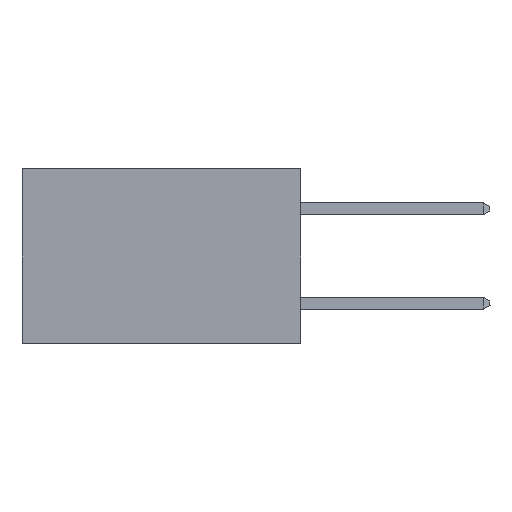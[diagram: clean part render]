
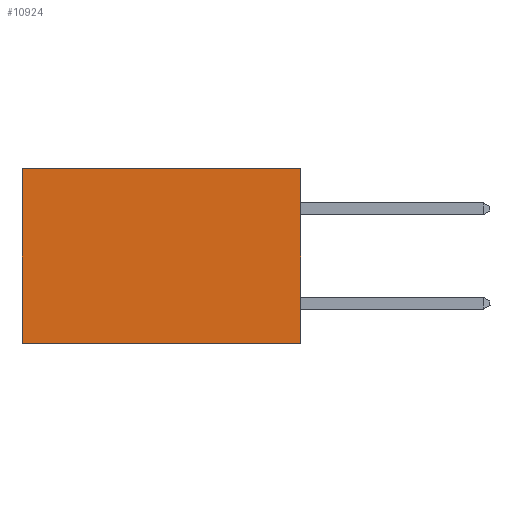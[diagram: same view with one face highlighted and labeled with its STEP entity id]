
A CAD part, left-side view. The second image highlights one B-rep face of the part: STEP entity #10924.
In plain terms, the highlighted planar face has unit normal (-1, 0, 0).
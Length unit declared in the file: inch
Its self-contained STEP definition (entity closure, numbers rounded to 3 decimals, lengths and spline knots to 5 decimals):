
#751 = LINE ( 'NONE', #3941, #12327 ) ;
#842 = EDGE_LOOP ( 'NONE', ( #27502, #11321, #12045, #11987 ) ) ;
#1211 = CARTESIAN_POINT ( 'NONE',  ( 0.277, 0.59, -0.37 ) ) ;
#2899 = DIRECTION ( 'NONE',  ( 0., 0., -1. ) ) ;
#3173 = CARTESIAN_POINT ( 'NONE',  ( 0.277, 0., 0. ) ) ;
#3523 = EDGE_CURVE ( 'NONE', #18295, #16183, #16042, .T. ) ;
#3941 = CARTESIAN_POINT ( 'NONE',  ( 0.277, 0., -0.37 ) ) ;
#4225 = DIRECTION ( 'NONE',  ( 0., 1., 0. ) ) ;
#4241 = DIRECTION ( 'NONE',  ( 0., 0., -1. ) ) ;
#5391 = VECTOR ( 'NONE', #5540, 39.37008 ) ;
#5540 = DIRECTION ( 'NONE',  ( 0., 1., 0. ) ) ;
#6784 = EDGE_CURVE ( 'NONE', #14167, #24368, #751, .T. ) ;
#8692 = PLANE ( 'NONE',  #21738 ) ;
#10018 = VECTOR ( 'NONE', #4225, 39.37008 ) ;
#10924 = ADVANCED_FACE ( 'NONE', ( #20927 ), #8692, .F. ) ;
#11009 = DIRECTION ( 'NONE',  ( 0., 0., -1. ) ) ;
#11321 = ORIENTED_EDGE ( 'NONE', *, *, #28337, .F. ) ;
#11987 = ORIENTED_EDGE ( 'NONE', *, *, #23821, .T. ) ;
#12045 = ORIENTED_EDGE ( 'NONE', *, *, #6784, .F. ) ;
#12327 = VECTOR ( 'NONE', #4241, 39.37008 ) ;
#12391 = CARTESIAN_POINT ( 'NONE',  ( 0.277, 0., -0.37 ) ) ;
#14167 = VERTEX_POINT ( 'NONE', #3173 ) ;
#15190 = CARTESIAN_POINT ( 'NONE',  ( 0.277, 0.59, 0. ) ) ;
#15632 = CARTESIAN_POINT ( 'NONE',  ( 0.277, 0., 0. ) ) ;
#16042 = LINE ( 'NONE', #1211, #20543 ) ;
#16183 = VERTEX_POINT ( 'NONE', #16940 ) ;
#16940 = CARTESIAN_POINT ( 'NONE',  ( 0.277, 0.59, -0.37 ) ) ;
#17332 = CARTESIAN_POINT ( 'NONE',  ( 0.277, 0., -0.37 ) ) ;
#18295 = VERTEX_POINT ( 'NONE', #15190 ) ;
#20543 = VECTOR ( 'NONE', #2899, 39.37008 ) ;
#20927 = FACE_OUTER_BOUND ( 'NONE', #842, .T. ) ;
#21738 = AXIS2_PLACEMENT_3D ( 'NONE', #22126, #24311, #11009 ) ;
#22126 = CARTESIAN_POINT ( 'NONE',  ( 0.277, 0., -0.37 ) ) ;
#23368 = LINE ( 'NONE', #12391, #5391 ) ;
#23821 = EDGE_CURVE ( 'NONE', #14167, #18295, #25669, .T. ) ;
#24311 = DIRECTION ( 'NONE',  ( 1., 0., 0. ) ) ;
#24368 = VERTEX_POINT ( 'NONE', #17332 ) ;
#25669 = LINE ( 'NONE', #15632, #10018 ) ;
#27502 = ORIENTED_EDGE ( 'NONE', *, *, #3523, .T. ) ;
#28337 = EDGE_CURVE ( 'NONE', #24368, #16183, #23368, .T. ) ;
